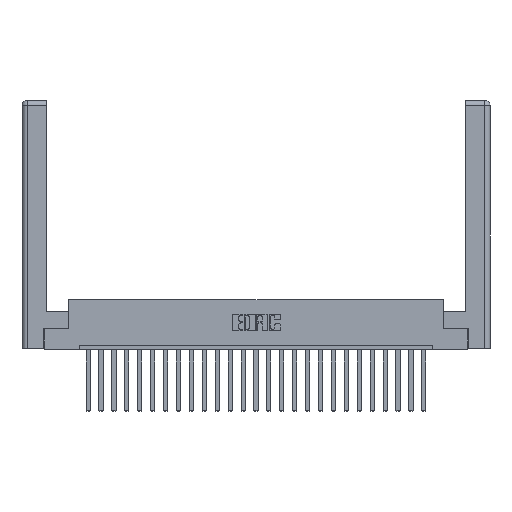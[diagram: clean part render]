
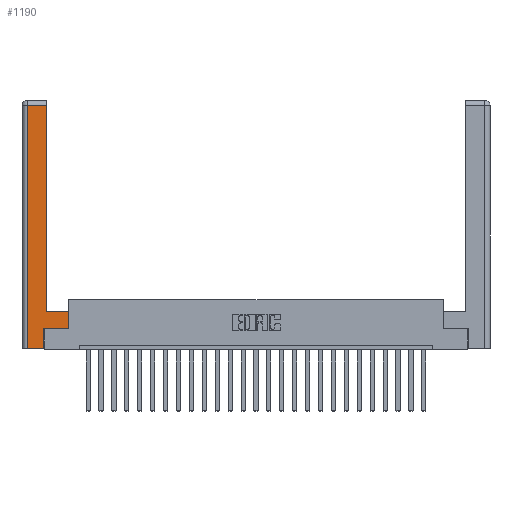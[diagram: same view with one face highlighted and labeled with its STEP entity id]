
A CAD part, top view. The second image highlights one B-rep face of the part: STEP entity #1190.
In plain terms, the highlighted planar face has unit normal (0, 0, 1).
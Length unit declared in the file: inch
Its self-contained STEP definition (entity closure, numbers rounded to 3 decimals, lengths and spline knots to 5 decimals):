
#31 = EDGE_CURVE ( 'NONE', #12776, #17694, #16786, .T. ) ;
#112 = CARTESIAN_POINT ( 'NONE',  ( 0.265, 0., 0. ) ) ;
#184 = DIRECTION ( 'NONE',  ( 0., 1., 0. ) ) ;
#412 = DIRECTION ( 'NONE',  ( -1., 0., 0. ) ) ;
#640 = VECTOR ( 'NONE', #5241, 39.37008 ) ;
#689 = ORIENTED_EDGE ( 'NONE', *, *, #6848, .T. ) ;
#1117 = DIRECTION ( 'NONE',  ( -1., 0., 0. ) ) ;
#1190 = ADVANCED_FACE ( 'NONE', ( #17615 ), #16930, .F. ) ;
#1799 = DIRECTION ( 'NONE',  ( 0., 0., -1. ) ) ;
#2364 = ORIENTED_EDGE ( 'NONE', *, *, #3416, .T. ) ;
#3256 = CARTESIAN_POINT ( 'NONE',  ( 0.295, 0.45, 0. ) ) ;
#3416 = EDGE_CURVE ( 'NONE', #18640, #8647, #4826, .T. ) ;
#4826 = LINE ( 'NONE', #10487, #7202 ) ;
#5241 = DIRECTION ( 'NONE',  ( 1., 0., 0. ) ) ;
#5291 = EDGE_CURVE ( 'NONE', #17694, #16507, #12418, .T. ) ;
#6620 = LINE ( 'NONE', #15538, #8096 ) ;
#6848 = EDGE_CURVE ( 'NONE', #7340, #18640, #7780, .T. ) ;
#7202 = VECTOR ( 'NONE', #1117, 39.37008 ) ;
#7241 = CARTESIAN_POINT ( 'NONE',  ( 0.0615, 2.94, 0. ) ) ;
#7340 = VERTEX_POINT ( 'NONE', #3256 ) ;
#7417 = ORIENTED_EDGE ( 'NONE', *, *, #15999, .T. ) ;
#7610 = CARTESIAN_POINT ( 'NONE',  ( 0.0615, 0., 0. ) ) ;
#7780 = LINE ( 'NONE', #17405, #19646 ) ;
#8096 = VECTOR ( 'NONE', #412, 39.37008 ) ;
#8647 = VERTEX_POINT ( 'NONE', #7241 ) ;
#9192 = DIRECTION ( 'NONE',  ( -1., 0., 0. ) ) ;
#9708 = LINE ( 'NONE', #7610, #21877 ) ;
#10106 = DIRECTION ( 'NONE',  ( 0., 1., 0. ) ) ;
#10248 = ORIENTED_EDGE ( 'NONE', *, *, #5291, .T. ) ;
#10487 = CARTESIAN_POINT ( 'NONE',  ( 0.0615, 2.94, 0. ) ) ;
#11135 = ORIENTED_EDGE ( 'NONE', *, *, #15417, .T. ) ;
#11383 = DIRECTION ( 'NONE',  ( 0., -1., 0. ) ) ;
#11956 = VERTEX_POINT ( 'NONE', #20490 ) ;
#12418 = LINE ( 'NONE', #20473, #640 ) ;
#12776 = VERTEX_POINT ( 'NONE', #18711 ) ;
#13860 = VECTOR ( 'NONE', #15113, 39.37008 ) ;
#14205 = ORIENTED_EDGE ( 'NONE', *, *, #21008, .T. ) ;
#14829 = EDGE_CURVE ( 'NONE', #11956, #12776, #21284, .T. ) ;
#15113 = DIRECTION ( 'NONE',  ( 0., 1., 0. ) ) ;
#15417 = EDGE_CURVE ( 'NONE', #16507, #23399, #18918, .T. ) ;
#15538 = CARTESIAN_POINT ( 'NONE',  ( 0.295, 0.45, 0. ) ) ;
#15728 = CARTESIAN_POINT ( 'NONE',  ( 0.265, 0.245, 0. ) ) ;
#15999 = EDGE_CURVE ( 'NONE', #8647, #11956, #9708, .T. ) ;
#16507 = VERTEX_POINT ( 'NONE', #21807 ) ;
#16786 = LINE ( 'NONE', #18542, #17695 ) ;
#16930 = PLANE ( 'NONE',  #17540 ) ;
#17097 = CARTESIAN_POINT ( 'NONE',  ( 0.565, 0.45, 0. ) ) ;
#17405 = CARTESIAN_POINT ( 'NONE',  ( 0.295, 3., 0. ) ) ;
#17540 = AXIS2_PLACEMENT_3D ( 'NONE', #18878, #1799, #9192 ) ;
#17615 = FACE_OUTER_BOUND ( 'NONE', #18795, .T. ) ;
#17694 = VERTEX_POINT ( 'NONE', #15728 ) ;
#17695 = VECTOR ( 'NONE', #10106, 39.37008 ) ;
#18315 = CARTESIAN_POINT ( 'NONE',  ( 0.565, 0.45, 0. ) ) ;
#18542 = CARTESIAN_POINT ( 'NONE',  ( 0.265, 0.245, 0. ) ) ;
#18634 = CARTESIAN_POINT ( 'NONE',  ( 0.295, 2.94, 0. ) ) ;
#18640 = VERTEX_POINT ( 'NONE', #18634 ) ;
#18711 = CARTESIAN_POINT ( 'NONE',  ( 0.265, 0., 0. ) ) ;
#18795 = EDGE_LOOP ( 'NONE', ( #689, #2364, #7417, #23235, #23512, #10248, #11135, #14205 ) ) ;
#18878 = CARTESIAN_POINT ( 'NONE',  ( 0., 0., 0. ) ) ;
#18918 = LINE ( 'NONE', #17097, #13860 ) ;
#19646 = VECTOR ( 'NONE', #184, 39.37008 ) ;
#19810 = VECTOR ( 'NONE', #22696, 39.37008 ) ;
#20473 = CARTESIAN_POINT ( 'NONE',  ( 0.565, 0.245, 0. ) ) ;
#20490 = CARTESIAN_POINT ( 'NONE',  ( 0.0615, 0., 0. ) ) ;
#21008 = EDGE_CURVE ( 'NONE', #23399, #7340, #6620, .T. ) ;
#21284 = LINE ( 'NONE', #112, #19810 ) ;
#21807 = CARTESIAN_POINT ( 'NONE',  ( 0.565, 0.245, 0. ) ) ;
#21877 = VECTOR ( 'NONE', #11383, 39.37008 ) ;
#22696 = DIRECTION ( 'NONE',  ( 1., 0., 0. ) ) ;
#23235 = ORIENTED_EDGE ( 'NONE', *, *, #14829, .T. ) ;
#23399 = VERTEX_POINT ( 'NONE', #18315 ) ;
#23512 = ORIENTED_EDGE ( 'NONE', *, *, #31, .T. ) ;
